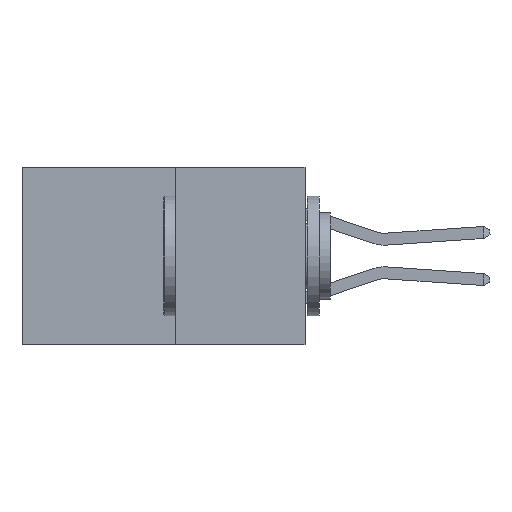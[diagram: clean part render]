
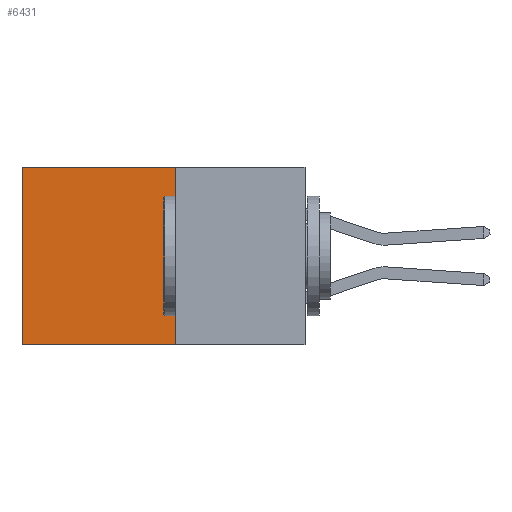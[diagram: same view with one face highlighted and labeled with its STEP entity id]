
A CAD part, left-side view. The second image highlights one B-rep face of the part: STEP entity #6431.
In plain terms, the highlighted planar face has unit normal (-1, 0, 0).
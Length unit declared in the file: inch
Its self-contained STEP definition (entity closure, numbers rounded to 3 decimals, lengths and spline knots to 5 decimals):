
#165 = EDGE_CURVE ( 'NONE', #10002, #9141, #4118, .T. ) ;
#456 = EDGE_CURVE ( 'NONE', #8305, #10002, #7248, .T. ) ;
#495 = EDGE_CURVE ( 'NONE', #8305, #8790, #8718, .T. ) ;
#558 = ORIENTED_EDGE ( 'NONE', *, *, #495, .T. ) ;
#1044 = VECTOR ( 'NONE', #9592, 39.37008 ) ;
#1430 = EDGE_CURVE ( 'NONE', #8790, #9141, #7368, .T. ) ;
#2480 = CARTESIAN_POINT ( 'NONE',  ( 0.277, 0.59, -0.37 ) ) ;
#3127 = CARTESIAN_POINT ( 'NONE',  ( 0.277, 0.27, -0.37 ) ) ;
#3509 = CARTESIAN_POINT ( 'NONE',  ( 0.277, 0.27, -0.37 ) ) ;
#3959 = CARTESIAN_POINT ( 'NONE',  ( 0.277, 0.27, 0. ) ) ;
#3969 = CARTESIAN_POINT ( 'NONE',  ( 0.277, 0.27, 0. ) ) ;
#4118 = LINE ( 'NONE', #3127, #8630 ) ;
#4293 = CARTESIAN_POINT ( 'NONE',  ( 0.277, 0.59, -0.37 ) ) ;
#4407 = CARTESIAN_POINT ( 'NONE',  ( 0.277, 0.27, -0.37 ) ) ;
#4567 = DIRECTION ( 'NONE',  ( 0., 0., -1. ) ) ;
#4582 = ORIENTED_EDGE ( 'NONE', *, *, #1430, .T. ) ;
#4648 = CARTESIAN_POINT ( 'NONE',  ( 0.277, 0.59, 0. ) ) ;
#5569 = DIRECTION ( 'NONE',  ( 0., 0., -1. ) ) ;
#5572 = DIRECTION ( 'NONE',  ( 1., 0., 0. ) ) ;
#5608 = CARTESIAN_POINT ( 'NONE',  ( 0.277, 0.27, -0.37 ) ) ;
#5640 = PLANE ( 'NONE',  #7022 ) ;
#5976 = DIRECTION ( 'NONE',  ( 0., 1., 0. ) ) ;
#6431 = ADVANCED_FACE ( 'NONE', ( #9105 ), #5640, .F. ) ;
#6654 = ORIENTED_EDGE ( 'NONE', *, *, #165, .F. ) ;
#6772 = VECTOR ( 'NONE', #5976, 39.37008 ) ;
#7022 = AXIS2_PLACEMENT_3D ( 'NONE', #5608, #5572, #5569 ) ;
#7248 = LINE ( 'NONE', #4407, #9173 ) ;
#7368 = LINE ( 'NONE', #2480, #1044 ) ;
#7479 = DIRECTION ( 'NONE',  ( 0., 1., 0. ) ) ;
#8305 = VERTEX_POINT ( 'NONE', #3959 ) ;
#8623 = ORIENTED_EDGE ( 'NONE', *, *, #456, .F. ) ;
#8630 = VECTOR ( 'NONE', #7479, 39.37008 ) ;
#8718 = LINE ( 'NONE', #3969, #6772 ) ;
#8790 = VERTEX_POINT ( 'NONE', #4648 ) ;
#9105 = FACE_OUTER_BOUND ( 'NONE', #9147, .T. ) ;
#9141 = VERTEX_POINT ( 'NONE', #4293 ) ;
#9147 = EDGE_LOOP ( 'NONE', ( #4582, #6654, #8623, #558 ) ) ;
#9173 = VECTOR ( 'NONE', #4567, 39.37008 ) ;
#9592 = DIRECTION ( 'NONE',  ( 0., 0., -1. ) ) ;
#10002 = VERTEX_POINT ( 'NONE', #3509 ) ;
